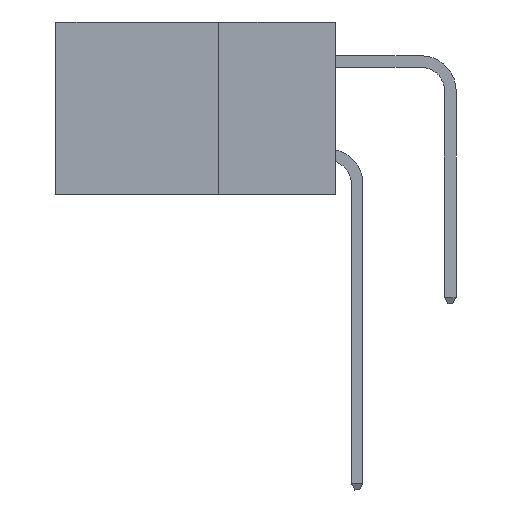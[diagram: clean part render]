
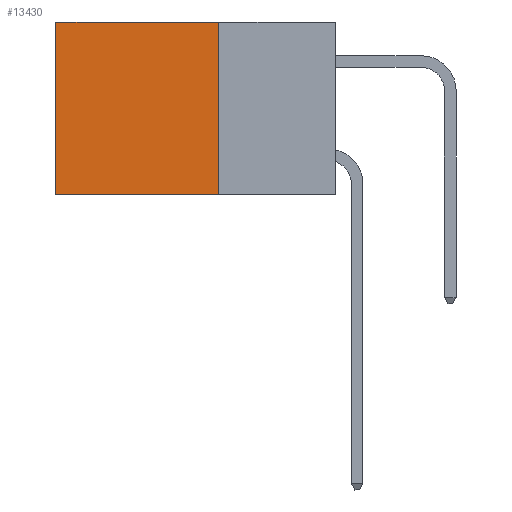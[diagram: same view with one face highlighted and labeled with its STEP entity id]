
A CAD part, left-side view. The second image highlights one B-rep face of the part: STEP entity #13430.
In plain terms, the highlighted planar face has unit normal (-1, 0, 0).
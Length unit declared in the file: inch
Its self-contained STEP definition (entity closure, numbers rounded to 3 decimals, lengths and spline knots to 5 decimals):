
#888 = VECTOR ( 'NONE', #8021, 39.37008 ) ;
#956 = ORIENTED_EDGE ( 'NONE', *, *, #2324, .F. ) ;
#1480 = EDGE_CURVE ( 'NONE', #10057, #11659, #11983, .T. ) ;
#2286 = VERTEX_POINT ( 'NONE', #9799 ) ;
#2324 = EDGE_CURVE ( 'NONE', #8410, #11659, #8323, .T. ) ;
#2355 = ORIENTED_EDGE ( 'NONE', *, *, #9457, .F. ) ;
#2532 = DIRECTION ( 'NONE',  ( 0., 1., 0. ) ) ;
#2602 = VECTOR ( 'NONE', #2532, 39.37008 ) ;
#2695 = CARTESIAN_POINT ( 'NONE',  ( 0.2875, 0.6, -0.37 ) ) ;
#2771 = ORIENTED_EDGE ( 'NONE', *, *, #1480, .T. ) ;
#3104 = EDGE_LOOP ( 'NONE', ( #2771, #956, #2355, #7096 ) ) ;
#3397 = CARTESIAN_POINT ( 'NONE',  ( 0.2875, 0.25, 0. ) ) ;
#3445 = CARTESIAN_POINT ( 'NONE',  ( 0.2875, 0.25, -0.37 ) ) ;
#4047 = LINE ( 'NONE', #9141, #888 ) ;
#4512 = CARTESIAN_POINT ( 'NONE',  ( 0.2875, 0.6, 0. ) ) ;
#4932 = AXIS2_PLACEMENT_3D ( 'NONE', #7974, #12524, #5708 ) ;
#5708 = DIRECTION ( 'NONE',  ( 0., 0., -1. ) ) ;
#7096 = ORIENTED_EDGE ( 'NONE', *, *, #11404, .T. ) ;
#7224 = VECTOR ( 'NONE', #10247, 39.37008 ) ;
#7548 = CARTESIAN_POINT ( 'NONE',  ( 0.2875, 0.6, 0. ) ) ;
#7573 = DIRECTION ( 'NONE',  ( 0., 0., -1. ) ) ;
#7682 = CARTESIAN_POINT ( 'NONE',  ( 0.2875, 0.25, -0.37 ) ) ;
#7974 = CARTESIAN_POINT ( 'NONE',  ( 0.2875, 0.25, 0. ) ) ;
#8021 = DIRECTION ( 'NONE',  ( 0., 0., -1. ) ) ;
#8253 = VECTOR ( 'NONE', #7573, 39.37008 ) ;
#8323 = LINE ( 'NONE', #3445, #2602 ) ;
#8410 = VERTEX_POINT ( 'NONE', #7682 ) ;
#9141 = CARTESIAN_POINT ( 'NONE',  ( 0.2875, 0.25, 0. ) ) ;
#9457 = EDGE_CURVE ( 'NONE', #2286, #8410, #4047, .T. ) ;
#9795 = FACE_OUTER_BOUND ( 'NONE', #3104, .T. ) ;
#9799 = CARTESIAN_POINT ( 'NONE',  ( 0.2875, 0.25, 0. ) ) ;
#10057 = VERTEX_POINT ( 'NONE', #4512 ) ;
#10178 = LINE ( 'NONE', #3397, #7224 ) ;
#10247 = DIRECTION ( 'NONE',  ( 0., 1., 0. ) ) ;
#11347 = PLANE ( 'NONE',  #4932 ) ;
#11404 = EDGE_CURVE ( 'NONE', #2286, #10057, #10178, .T. ) ;
#11659 = VERTEX_POINT ( 'NONE', #2695 ) ;
#11983 = LINE ( 'NONE', #7548, #8253 ) ;
#12524 = DIRECTION ( 'NONE',  ( 1., 0., 0. ) ) ;
#13430 = ADVANCED_FACE ( 'NONE', ( #9795 ), #11347, .F. ) ;
